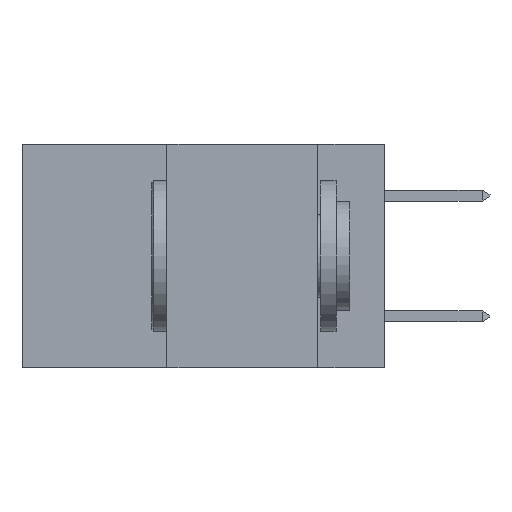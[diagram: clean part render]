
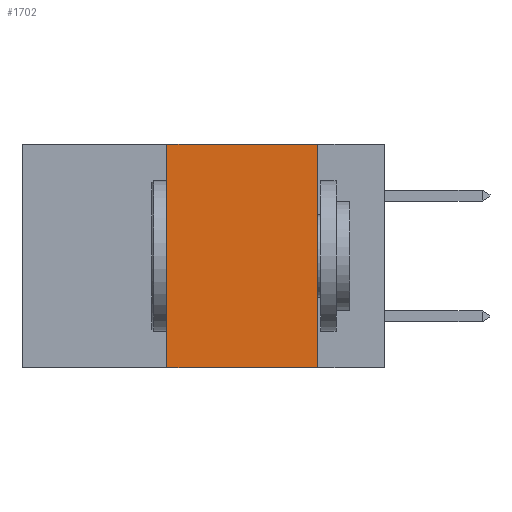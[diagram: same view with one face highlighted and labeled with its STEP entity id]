
A CAD part, left-side view. The second image highlights one B-rep face of the part: STEP entity #1702.
In plain terms, the highlighted planar face has unit normal (-1, 0, 0).
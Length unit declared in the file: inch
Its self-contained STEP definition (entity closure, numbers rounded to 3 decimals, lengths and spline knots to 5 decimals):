
#802 = LINE ( 'NONE', #1637, #5975 ) ;
#936 = DIRECTION ( 'NONE',  ( 0., 0., -1. ) ) ;
#1433 = ORIENTED_EDGE ( 'NONE', *, *, #3670, .F. ) ;
#1637 = CARTESIAN_POINT ( 'NONE',  ( 0., 0.36, 0. ) ) ;
#1646 = DIRECTION ( 'NONE',  ( 0., 0., 1. ) ) ;
#1702 = ADVANCED_FACE ( 'NONE', ( #11863 ), #11689, .F. ) ;
#2486 = VECTOR ( 'NONE', #6401, 39.37008 ) ;
#2596 = LINE ( 'NONE', #8083, #5607 ) ;
#3044 = VECTOR ( 'NONE', #12075, 39.37008 ) ;
#3225 = EDGE_CURVE ( 'NONE', #11262, #4185, #5686, .T. ) ;
#3670 = EDGE_CURVE ( 'NONE', #11262, #5659, #802, .T. ) ;
#4185 = VERTEX_POINT ( 'NONE', #8228 ) ;
#4382 = EDGE_CURVE ( 'NONE', #5659, #9451, #8413, .T. ) ;
#4813 = DIRECTION ( 'NONE',  ( 1., 0., 0. ) ) ;
#5607 = VECTOR ( 'NONE', #936, 39.37008 ) ;
#5659 = VERTEX_POINT ( 'NONE', #9823 ) ;
#5679 = EDGE_LOOP ( 'NONE', ( #10430, #12391, #1433, #6494 ) ) ;
#5686 = LINE ( 'NONE', #12610, #3044 ) ;
#5975 = VECTOR ( 'NONE', #1646, 39.37008 ) ;
#6401 = DIRECTION ( 'NONE',  ( 0., -1., 0. ) ) ;
#6418 = CARTESIAN_POINT ( 'NONE',  ( 0., 0.6, 0. ) ) ;
#6494 = ORIENTED_EDGE ( 'NONE', *, *, #3225, .T. ) ;
#7244 = CARTESIAN_POINT ( 'NONE',  ( 0., 0.36, -0.37 ) ) ;
#7828 = AXIS2_PLACEMENT_3D ( 'NONE', #11899, #4813, #11639 ) ;
#8083 = CARTESIAN_POINT ( 'NONE',  ( 0., 0.11, 0. ) ) ;
#8228 = CARTESIAN_POINT ( 'NONE',  ( 0., 0.11, -0.37 ) ) ;
#8413 = LINE ( 'NONE', #6418, #2486 ) ;
#9451 = VERTEX_POINT ( 'NONE', #10688 ) ;
#9823 = CARTESIAN_POINT ( 'NONE',  ( 0., 0.36, 0. ) ) ;
#10237 = EDGE_CURVE ( 'NONE', #9451, #4185, #2596, .T. ) ;
#10430 = ORIENTED_EDGE ( 'NONE', *, *, #10237, .F. ) ;
#10688 = CARTESIAN_POINT ( 'NONE',  ( 0., 0.11, 0. ) ) ;
#11262 = VERTEX_POINT ( 'NONE', #7244 ) ;
#11639 = DIRECTION ( 'NONE',  ( 0., 0., -1. ) ) ;
#11689 = PLANE ( 'NONE',  #7828 ) ;
#11863 = FACE_OUTER_BOUND ( 'NONE', #5679, .T. ) ;
#11899 = CARTESIAN_POINT ( 'NONE',  ( 0., 0.6, 0. ) ) ;
#12075 = DIRECTION ( 'NONE',  ( 0., -1., 0. ) ) ;
#12391 = ORIENTED_EDGE ( 'NONE', *, *, #4382, .F. ) ;
#12610 = CARTESIAN_POINT ( 'NONE',  ( 0., 0.6, -0.37 ) ) ;
